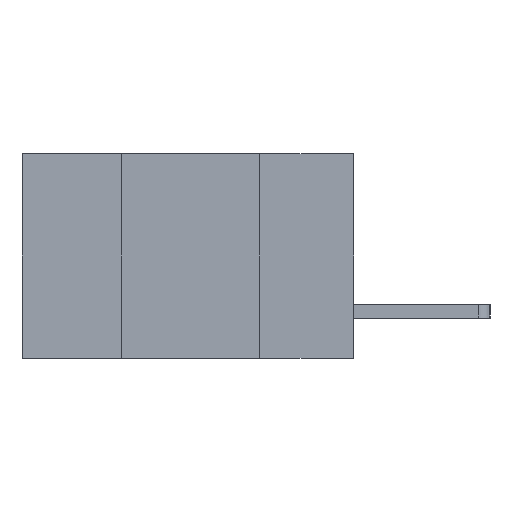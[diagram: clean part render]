
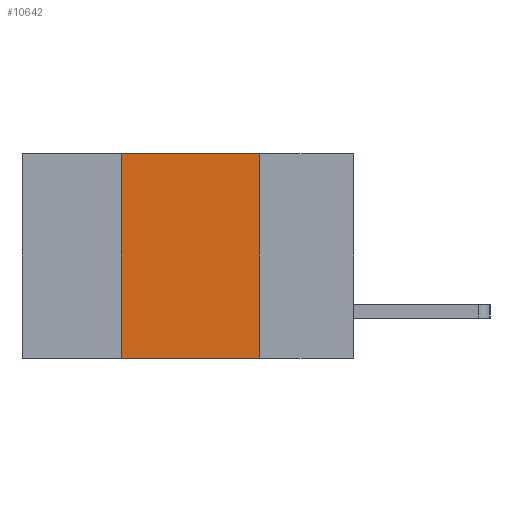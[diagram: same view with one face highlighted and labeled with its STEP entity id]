
A CAD part, left-side view. The second image highlights one B-rep face of the part: STEP entity #10642.
In plain terms, the highlighted planar face has unit normal (-1, 0, 0).
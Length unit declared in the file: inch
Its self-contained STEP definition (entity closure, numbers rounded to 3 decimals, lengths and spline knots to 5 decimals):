
#446 = LINE ( 'NONE', #4942, #8203 ) ;
#1016 = VECTOR ( 'NONE', #6444, 39.37008 ) ;
#1057 = CARTESIAN_POINT ( 'NONE',  ( 0., 0.42, -0.37 ) ) ;
#1091 = EDGE_CURVE ( 'NONE', #13110, #12133, #4668, .T. ) ;
#1235 = DIRECTION ( 'NONE',  ( 1., 0., 0. ) ) ;
#1296 = CARTESIAN_POINT ( 'NONE',  ( 0., 0.6, 0. ) ) ;
#1366 = LINE ( 'NONE', #11350, #6656 ) ;
#2066 = VERTEX_POINT ( 'NONE', #11700 ) ;
#2232 = EDGE_CURVE ( 'NONE', #3296, #12133, #5518, .T. ) ;
#2520 = CARTESIAN_POINT ( 'NONE',  ( 0., 0.17, 0. ) ) ;
#3188 = DIRECTION ( 'NONE',  ( 0., -1., 0. ) ) ;
#3296 = VERTEX_POINT ( 'NONE', #2520 ) ;
#4668 = LINE ( 'NONE', #8520, #12037 ) ;
#4671 = ORIENTED_EDGE ( 'NONE', *, *, #10984, .F. ) ;
#4942 = CARTESIAN_POINT ( 'NONE',  ( 0., 0.42, 0. ) ) ;
#5518 = LINE ( 'NONE', #6517, #1016 ) ;
#6385 = PLANE ( 'NONE',  #7484 ) ;
#6444 = DIRECTION ( 'NONE',  ( 0., 0., -1. ) ) ;
#6517 = CARTESIAN_POINT ( 'NONE',  ( 0., 0.17, 0. ) ) ;
#6656 = VECTOR ( 'NONE', #3188, 39.37008 ) ;
#7484 = AXIS2_PLACEMENT_3D ( 'NONE', #1296, #1235, #9502 ) ;
#8203 = VECTOR ( 'NONE', #10967, 39.37008 ) ;
#8520 = CARTESIAN_POINT ( 'NONE',  ( 0., 0.6, -0.37 ) ) ;
#9229 = EDGE_LOOP ( 'NONE', ( #9296, #4671, #10170, #10498 ) ) ;
#9296 = ORIENTED_EDGE ( 'NONE', *, *, #2232, .F. ) ;
#9502 = DIRECTION ( 'NONE',  ( 0., 0., -1. ) ) ;
#10170 = ORIENTED_EDGE ( 'NONE', *, *, #12242, .F. ) ;
#10498 = ORIENTED_EDGE ( 'NONE', *, *, #1091, .T. ) ;
#10642 = ADVANCED_FACE ( 'NONE', ( #12338 ), #6385, .F. ) ;
#10967 = DIRECTION ( 'NONE',  ( 0., 0., 1. ) ) ;
#10984 = EDGE_CURVE ( 'NONE', #2066, #3296, #1366, .T. ) ;
#11350 = CARTESIAN_POINT ( 'NONE',  ( 0., 0.6, 0. ) ) ;
#11700 = CARTESIAN_POINT ( 'NONE',  ( 0., 0.42, 0. ) ) ;
#12037 = VECTOR ( 'NONE', #12746, 39.37008 ) ;
#12133 = VERTEX_POINT ( 'NONE', #12630 ) ;
#12242 = EDGE_CURVE ( 'NONE', #13110, #2066, #446, .T. ) ;
#12338 = FACE_OUTER_BOUND ( 'NONE', #9229, .T. ) ;
#12630 = CARTESIAN_POINT ( 'NONE',  ( 0., 0.17, -0.37 ) ) ;
#12746 = DIRECTION ( 'NONE',  ( 0., -1., 0. ) ) ;
#13110 = VERTEX_POINT ( 'NONE', #1057 ) ;
